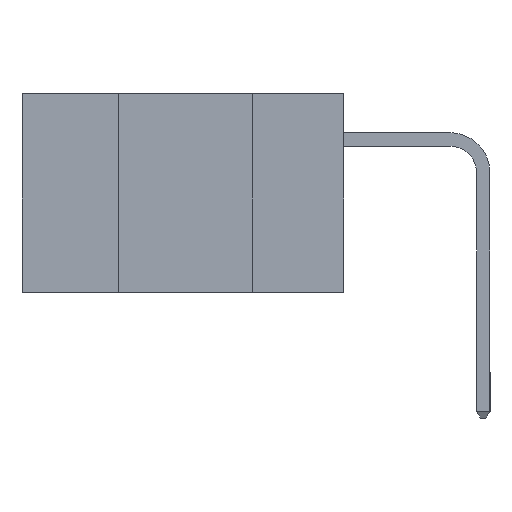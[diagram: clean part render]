
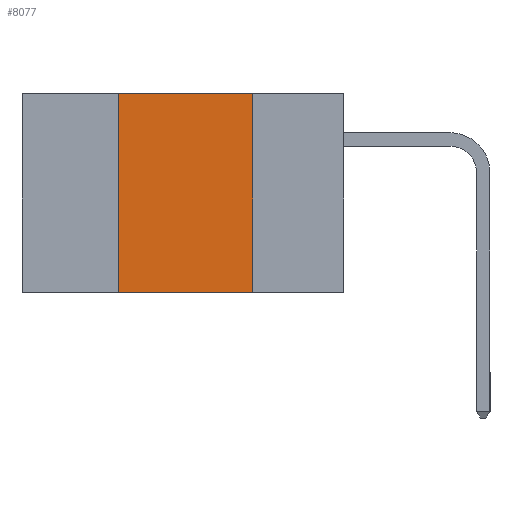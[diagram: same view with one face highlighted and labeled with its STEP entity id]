
A CAD part, left-side view. The second image highlights one B-rep face of the part: STEP entity #8077.
In plain terms, the highlighted planar face has unit normal (-1, 0, 0).
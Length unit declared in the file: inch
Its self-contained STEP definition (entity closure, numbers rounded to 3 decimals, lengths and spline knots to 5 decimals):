
#449 = EDGE_CURVE ( 'NONE', #6690, #2391, #5443, .T. ) ;
#586 = CARTESIAN_POINT ( 'NONE',  ( 0., 0.17, 0. ) ) ;
#1272 = EDGE_CURVE ( 'NONE', #2391, #6973, #3274, .T. ) ;
#2377 = DIRECTION ( 'NONE',  ( 0., -1., 0. ) ) ;
#2391 = VERTEX_POINT ( 'NONE', #586 ) ;
#2427 = DIRECTION ( 'NONE',  ( 0., -1., 0. ) ) ;
#2477 = CARTESIAN_POINT ( 'NONE',  ( 0., 0.42, 0. ) ) ;
#2543 = DIRECTION ( 'NONE',  ( 0., 0., -1. ) ) ;
#2671 = ORIENTED_EDGE ( 'NONE', *, *, #449, .F. ) ;
#2698 = AXIS2_PLACEMENT_3D ( 'NONE', #6190, #6292, #4035 ) ;
#3067 = VECTOR ( 'NONE', #3526, 39.37008 ) ;
#3069 = CARTESIAN_POINT ( 'NONE',  ( 0., 0.17, -0.37 ) ) ;
#3098 = CARTESIAN_POINT ( 'NONE',  ( 0., 0.6, -0.37 ) ) ;
#3274 = LINE ( 'NONE', #3069, #9209 ) ;
#3377 = FACE_OUTER_BOUND ( 'NONE', #9000, .T. ) ;
#3526 = DIRECTION ( 'NONE',  ( 0., 0., 1. ) ) ;
#4035 = DIRECTION ( 'NONE',  ( 0., 0., -1. ) ) ;
#4083 = PLANE ( 'NONE',  #2698 ) ;
#4182 = ORIENTED_EDGE ( 'NONE', *, *, #4563, .T. ) ;
#4232 = LINE ( 'NONE', #7179, #3067 ) ;
#4534 = ORIENTED_EDGE ( 'NONE', *, *, #5795, .F. ) ;
#4563 = EDGE_CURVE ( 'NONE', #5833, #6973, #6757, .T. ) ;
#4628 = CARTESIAN_POINT ( 'NONE',  ( 0., 0.42, -0.37 ) ) ;
#4937 = ORIENTED_EDGE ( 'NONE', *, *, #1272, .F. ) ;
#5443 = LINE ( 'NONE', #9188, #5938 ) ;
#5795 = EDGE_CURVE ( 'NONE', #5833, #6690, #4232, .T. ) ;
#5833 = VERTEX_POINT ( 'NONE', #4628 ) ;
#5938 = VECTOR ( 'NONE', #2427, 39.37008 ) ;
#6190 = CARTESIAN_POINT ( 'NONE',  ( 0., 0.6, 0. ) ) ;
#6292 = DIRECTION ( 'NONE',  ( 1., 0., 0. ) ) ;
#6690 = VERTEX_POINT ( 'NONE', #2477 ) ;
#6757 = LINE ( 'NONE', #3098, #8570 ) ;
#6973 = VERTEX_POINT ( 'NONE', #9526 ) ;
#7179 = CARTESIAN_POINT ( 'NONE',  ( 0., 0.42, -0.37 ) ) ;
#8077 = ADVANCED_FACE ( 'NONE', ( #3377 ), #4083, .F. ) ;
#8570 = VECTOR ( 'NONE', #2377, 39.37008 ) ;
#9000 = EDGE_LOOP ( 'NONE', ( #4937, #2671, #4534, #4182 ) ) ;
#9188 = CARTESIAN_POINT ( 'NONE',  ( 0., 0.6, 0. ) ) ;
#9209 = VECTOR ( 'NONE', #2543, 39.37008 ) ;
#9526 = CARTESIAN_POINT ( 'NONE',  ( 0., 0.17, -0.37 ) ) ;
